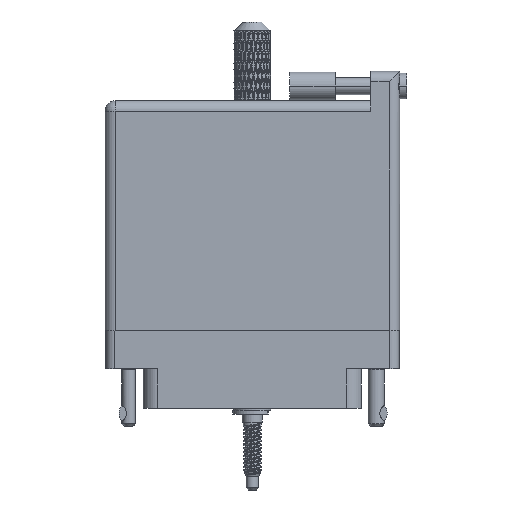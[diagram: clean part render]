
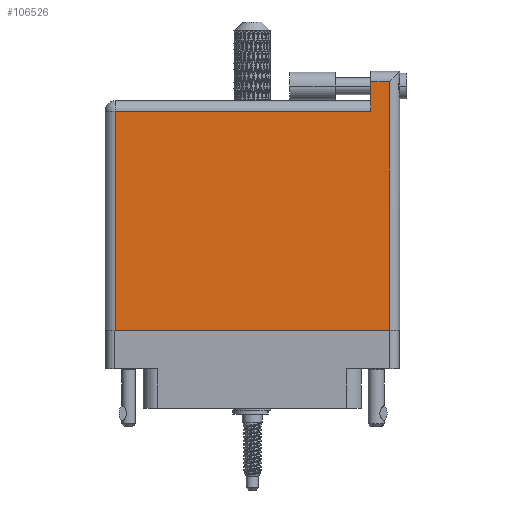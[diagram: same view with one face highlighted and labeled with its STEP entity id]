
A CAD part, front view. The second image highlights one B-rep face of the part: STEP entity #106526.
In plain terms, the highlighted face is planar.
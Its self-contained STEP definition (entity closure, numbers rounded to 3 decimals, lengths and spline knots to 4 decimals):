
#182 = CARTESIAN_POINT ( 'NONE',  ( 1.811, 1.766, 0. ) ) ;
#2495 = CARTESIAN_POINT ( 'NONE',  ( 0.07, 0., 0. ) ) ;
#5208 = EDGE_CURVE ( 'NONE', #98700, #89823, #16740, .T. ) ;
#8738 = CARTESIAN_POINT ( 'NONE',  ( 1.811, 1.696, 0. ) ) ;
#9737 = ORIENTED_EDGE ( 'NONE', *, *, #100204, .T. ) ;
#11637 = DIRECTION ( 'NONE',  ( 0., -1., 0. ) ) ;
#14925 = LINE ( 'NONE', #22926, #105657 ) ;
#16740 = LINE ( 'NONE', #2495, #110068 ) ;
#22926 = CARTESIAN_POINT ( 'NONE',  ( 0., 0., 0. ) ) ;
#23095 = EDGE_CURVE ( 'NONE', #57355, #88823, #102390, .T. ) ;
#24617 = ORIENTED_EDGE ( 'NONE', *, *, #109369, .T. ) ;
#25774 = LINE ( 'NONE', #182, #75258 ) ;
#25885 = ORIENTED_EDGE ( 'NONE', *, *, #93230, .T. ) ;
#26543 = DIRECTION ( 'NONE',  ( -1., 0., 0. ) ) ;
#30852 = LINE ( 'NONE', #79222, #96866 ) ;
#32015 = AXIS2_PLACEMENT_3D ( 'NONE', #89518, #64206, #100999 ) ;
#36814 = CARTESIAN_POINT ( 'NONE',  ( 1.938, 0., 0. ) ) ;
#39646 = PLANE ( 'NONE',  #32015 ) ;
#41435 = DIRECTION ( 'NONE',  ( 1., 0., 0. ) ) ;
#43563 = DIRECTION ( 'NONE',  ( 0., -1., 0. ) ) ;
#43972 = ORIENTED_EDGE ( 'NONE', *, *, #23095, .T. ) ;
#45434 = CARTESIAN_POINT ( 'NONE',  ( 0.07, 1.496, 0. ) ) ;
#45668 = CARTESIAN_POINT ( 'NONE',  ( 0.07, 0., 0. ) ) ;
#52605 = ORIENTED_EDGE ( 'NONE', *, *, #5208, .T. ) ;
#55273 = CARTESIAN_POINT ( 'NONE',  ( 1.938, 1.766, 0. ) ) ;
#57355 = VERTEX_POINT ( 'NONE', #102110 ) ;
#61939 = EDGE_LOOP ( 'NONE', ( #9737, #24617, #43972, #67734, #25885, #52605 ) ) ;
#62050 = CARTESIAN_POINT ( 'NONE',  ( 1.811, 1.496, 0. ) ) ;
#64206 = DIRECTION ( 'NONE',  ( 0., 0., -1. ) ) ;
#65391 = VERTEX_POINT ( 'NONE', #36814 ) ;
#66248 = FACE_OUTER_BOUND ( 'NONE', #61939, .T. ) ;
#67734 = ORIENTED_EDGE ( 'NONE', *, *, #85543, .T. ) ;
#68364 = VECTOR ( 'NONE', #72157, 39.3701 ) ;
#72157 = DIRECTION ( 'NONE',  ( 0., 1., 0. ) ) ;
#75004 = DIRECTION ( 'NONE',  ( -1., 0., 0. ) ) ;
#75258 = VECTOR ( 'NONE', #43563, 39.3701 ) ;
#79119 = VECTOR ( 'NONE', #75004, 39.3701 ) ;
#79222 = CARTESIAN_POINT ( 'NONE',  ( 0., 1.496, 0. ) ) ;
#85543 = EDGE_CURVE ( 'NONE', #88823, #107055, #25774, .T. ) ;
#88823 = VERTEX_POINT ( 'NONE', #8738 ) ;
#89518 = CARTESIAN_POINT ( 'NONE',  ( 0., 1.566, 0. ) ) ;
#89823 = VERTEX_POINT ( 'NONE', #45668 ) ;
#93230 = EDGE_CURVE ( 'NONE', #107055, #98700, #30852, .T. ) ;
#96866 = VECTOR ( 'NONE', #26543, 39.3701 ) ;
#98700 = VERTEX_POINT ( 'NONE', #45434 ) ;
#100204 = EDGE_CURVE ( 'NONE', #89823, #65391, #14925, .T. ) ;
#100999 = DIRECTION ( 'NONE',  ( -1., 0., 0. ) ) ;
#102110 = CARTESIAN_POINT ( 'NONE',  ( 1.938, 1.696, 0. ) ) ;
#102213 = CARTESIAN_POINT ( 'NONE',  ( 0., 1.696, 0. ) ) ;
#102390 = LINE ( 'NONE', #102213, #79119 ) ;
#105657 = VECTOR ( 'NONE', #41435, 39.3701 ) ;
#106526 = ADVANCED_FACE ( 'NONE', ( #66248 ), #39646, .F. ) ;
#107055 = VERTEX_POINT ( 'NONE', #62050 ) ;
#109369 = EDGE_CURVE ( 'NONE', #65391, #57355, #112246, .T. ) ;
#110068 = VECTOR ( 'NONE', #11637, 39.3701 ) ;
#112246 = LINE ( 'NONE', #55273, #68364 ) ;
